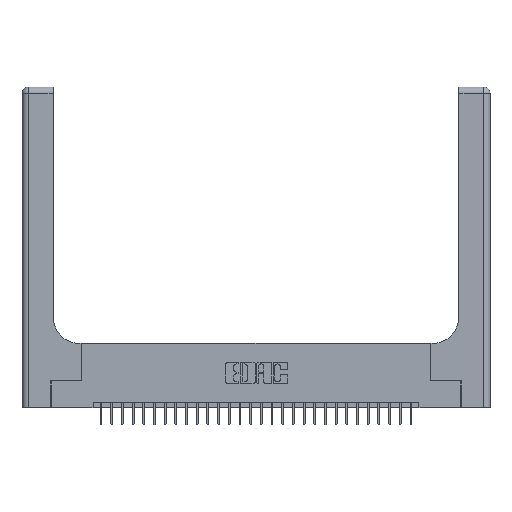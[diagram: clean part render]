
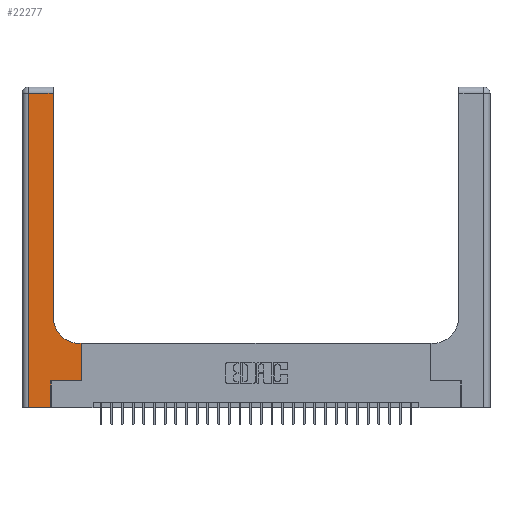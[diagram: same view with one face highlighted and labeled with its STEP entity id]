
A CAD part, top view. The second image highlights one B-rep face of the part: STEP entity #22277.
In plain terms, the highlighted planar face has unit normal (0, 0, 1).
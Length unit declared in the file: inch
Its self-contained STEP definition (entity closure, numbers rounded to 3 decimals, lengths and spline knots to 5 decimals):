
#217 = DIRECTION ( 'NONE',  ( 1., 0., 0. ) ) ;
#401 = VERTEX_POINT ( 'NONE', #19087 ) ;
#899 = VERTEX_POINT ( 'NONE', #4601 ) ;
#1616 = ORIENTED_EDGE ( 'NONE', *, *, #19050, .T. ) ;
#2556 = PLANE ( 'NONE',  #5355 ) ;
#2583 = ORIENTED_EDGE ( 'NONE', *, *, #10547, .T. ) ;
#2855 = VECTOR ( 'NONE', #3615, 39.37008 ) ;
#2859 = AXIS2_PLACEMENT_3D ( 'NONE', #9850, #26139, #12232 ) ;
#3615 = DIRECTION ( 'NONE',  ( -1., 0., 0. ) ) ;
#3746 = EDGE_CURVE ( 'NONE', #401, #5413, #28487, .T. ) ;
#4601 = CARTESIAN_POINT ( 'NONE',  ( 0.5415, 0.6, 0.37 ) ) ;
#4837 = CARTESIAN_POINT ( 'NONE',  ( 0., 2.94, 0.37 ) ) ;
#5097 = CARTESIAN_POINT ( 'NONE',  ( 0.269, 0.25, 0.37 ) ) ;
#5355 = AXIS2_PLACEMENT_3D ( 'NONE', #23736, #9752, #26038 ) ;
#5411 = VERTEX_POINT ( 'NONE', #20342 ) ;
#5413 = VERTEX_POINT ( 'NONE', #22672 ) ;
#5641 = CARTESIAN_POINT ( 'NONE',  ( 0.269, 0., 0.37 ) ) ;
#6364 = VERTEX_POINT ( 'NONE', #10455 ) ;
#6675 = CARTESIAN_POINT ( 'NONE',  ( 0.269, 0., 0.37 ) ) ;
#6756 = ORIENTED_EDGE ( 'NONE', *, *, #8187, .T. ) ;
#7719 = DIRECTION ( 'NONE',  ( 0., 1., 0. ) ) ;
#7823 = VERTEX_POINT ( 'NONE', #18296 ) ;
#7855 = VERTEX_POINT ( 'NONE', #23345 ) ;
#8187 = EDGE_CURVE ( 'NONE', #7823, #6364, #20569, .T. ) ;
#8413 = EDGE_CURVE ( 'NONE', #5413, #899, #21649, .T. ) ;
#8762 = ORIENTED_EDGE ( 'NONE', *, *, #3746, .T. ) ;
#8834 = VECTOR ( 'NONE', #7719, 39.37008 ) ;
#9083 = DIRECTION ( 'NONE',  ( 0., 1., 0. ) ) ;
#9528 = LINE ( 'NONE', #19883, #21210 ) ;
#9752 = DIRECTION ( 'NONE',  ( 0., 0., -1. ) ) ;
#9850 = CARTESIAN_POINT ( 'NONE',  ( 0.5415, 0.85, 0.37 ) ) ;
#10455 = CARTESIAN_POINT ( 'NONE',  ( 0.2915, 2.94, 0.37 ) ) ;
#10541 = EDGE_CURVE ( 'NONE', #7855, #13206, #21142, .T. ) ;
#10547 = EDGE_CURVE ( 'NONE', #13577, #401, #27295, .T. ) ;
#12209 = CARTESIAN_POINT ( 'NONE',  ( 0.5585, 0.25, 0.37 ) ) ;
#12232 = DIRECTION ( 'NONE',  ( 1., 0., 0. ) ) ;
#13206 = VERTEX_POINT ( 'NONE', #5641 ) ;
#13577 = VERTEX_POINT ( 'NONE', #23566 ) ;
#14993 = VECTOR ( 'NONE', #217, 39.37008 ) ;
#17272 = ORIENTED_EDGE ( 'NONE', *, *, #10541, .T. ) ;
#17749 = ORIENTED_EDGE ( 'NONE', *, *, #22847, .T. ) ;
#18296 = CARTESIAN_POINT ( 'NONE',  ( 0.2915, 0.85, 0.37 ) ) ;
#19050 = EDGE_CURVE ( 'NONE', #899, #7823, #19609, .T. ) ;
#19087 = CARTESIAN_POINT ( 'NONE',  ( 0.5585, 0.25, 0.37 ) ) ;
#19609 = CIRCLE ( 'NONE', #2859, 0.25 ) ;
#19883 = CARTESIAN_POINT ( 'NONE',  ( 0.06, 3., 0.37 ) ) ;
#19896 = VECTOR ( 'NONE', #9083, 39.37008 ) ;
#20342 = CARTESIAN_POINT ( 'NONE',  ( 0.06, 2.94, 0.37 ) ) ;
#20569 = LINE ( 'NONE', #21749, #8834 ) ;
#20611 = LINE ( 'NONE', #6675, #19896 ) ;
#21142 = LINE ( 'NONE', #28385, #14993 ) ;
#21210 = VECTOR ( 'NONE', #24504, 39.37008 ) ;
#21273 = DIRECTION ( 'NONE',  ( -1., 0., 0. ) ) ;
#21649 = LINE ( 'NONE', #29403, #2855 ) ;
#21749 = CARTESIAN_POINT ( 'NONE',  ( 0.2915, 3., 0.37 ) ) ;
#22277 = ADVANCED_FACE ( 'NONE', ( #26295 ), #2556, .F. ) ;
#22332 = VECTOR ( 'NONE', #28558, 39.37008 ) ;
#22365 = EDGE_LOOP ( 'NONE', ( #6756, #17749, #26254, #17272, #23695, #2583, #8762, #28187, #1616 ) ) ;
#22484 = EDGE_CURVE ( 'NONE', #5411, #7855, #9528, .T. ) ;
#22672 = CARTESIAN_POINT ( 'NONE',  ( 0.5585, 0.6, 0.37 ) ) ;
#22847 = EDGE_CURVE ( 'NONE', #6364, #5411, #24787, .T. ) ;
#23345 = CARTESIAN_POINT ( 'NONE',  ( 0.06, 0., 0.37 ) ) ;
#23566 = CARTESIAN_POINT ( 'NONE',  ( 0.269, 0.25, 0.37 ) ) ;
#23695 = ORIENTED_EDGE ( 'NONE', *, *, #29300, .T. ) ;
#23736 = CARTESIAN_POINT ( 'NONE',  ( 0., 3., 0.37 ) ) ;
#24504 = DIRECTION ( 'NONE',  ( 0., -1., 0. ) ) ;
#24787 = LINE ( 'NONE', #4837, #30228 ) ;
#26038 = DIRECTION ( 'NONE',  ( -1., 0., 0. ) ) ;
#26050 = DIRECTION ( 'NONE',  ( 1., 0., 0. ) ) ;
#26139 = DIRECTION ( 'NONE',  ( 0., 0., -1. ) ) ;
#26254 = ORIENTED_EDGE ( 'NONE', *, *, #22484, .T. ) ;
#26295 = FACE_OUTER_BOUND ( 'NONE', #22365, .T. ) ;
#26573 = VECTOR ( 'NONE', #26050, 39.37008 ) ;
#27295 = LINE ( 'NONE', #5097, #26573 ) ;
#28187 = ORIENTED_EDGE ( 'NONE', *, *, #8413, .T. ) ;
#28385 = CARTESIAN_POINT ( 'NONE',  ( 0., 0., 0.37 ) ) ;
#28487 = LINE ( 'NONE', #12209, #22332 ) ;
#28558 = DIRECTION ( 'NONE',  ( 0., 1., 0. ) ) ;
#29300 = EDGE_CURVE ( 'NONE', #13206, #13577, #20611, .T. ) ;
#29403 = CARTESIAN_POINT ( 'NONE',  ( 0.2915, 0.6, 0.37 ) ) ;
#30228 = VECTOR ( 'NONE', #21273, 39.37008 ) ;
